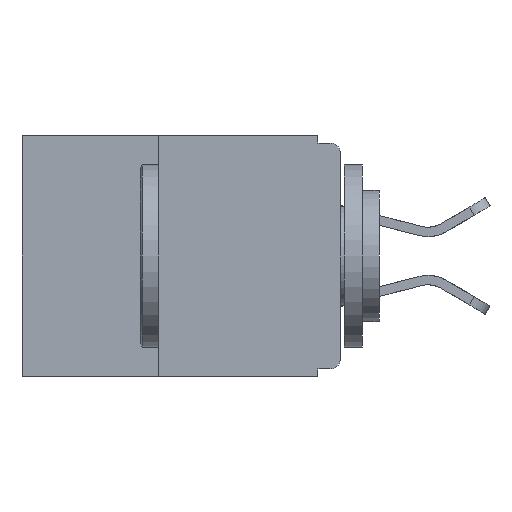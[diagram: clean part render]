
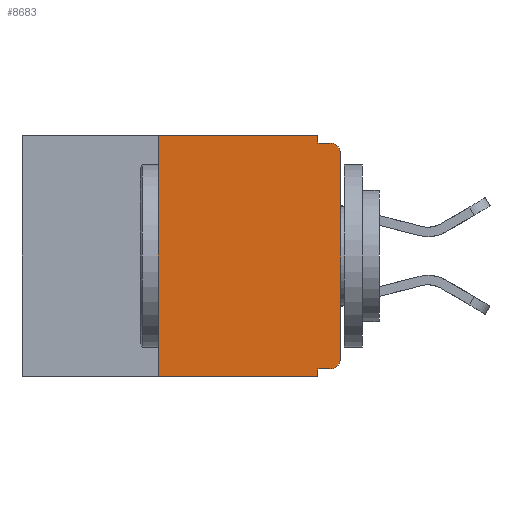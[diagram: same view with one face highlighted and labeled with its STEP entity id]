
A CAD part, left-side view. The second image highlights one B-rep face of the part: STEP entity #8683.
In plain terms, the highlighted planar face has unit normal (-1, 0, 0).
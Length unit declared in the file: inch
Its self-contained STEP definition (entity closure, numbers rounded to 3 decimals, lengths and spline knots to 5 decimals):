
#528 = EDGE_LOOP ( 'NONE', ( #21053, #15712, #7214, #2665, #1488, #900, #3362, #13361, #14241, #6404 ) ) ;
#668 = CARTESIAN_POINT ( 'NONE',  ( 0., 0.437, 0. ) ) ;
#900 = ORIENTED_EDGE ( 'NONE', *, *, #15830, .F. ) ;
#923 = EDGE_CURVE ( 'NONE', #12064, #20988, #22209, .T. ) ;
#1138 = CARTESIAN_POINT ( 'NONE',  ( 0., 0.031, -0.33 ) ) ;
#1488 = ORIENTED_EDGE ( 'NONE', *, *, #19813, .F. ) ;
#2294 = CARTESIAN_POINT ( 'NONE',  ( 0., 0., 0. ) ) ;
#2553 = PLANE ( 'NONE',  #15435 ) ;
#2558 = CARTESIAN_POINT ( 'NONE',  ( 0., 0.437, -0.33 ) ) ;
#2665 = ORIENTED_EDGE ( 'NONE', *, *, #14921, .F. ) ;
#2700 = DIRECTION ( 'NONE',  ( 0., 1., 0. ) ) ;
#2914 = EDGE_CURVE ( 'NONE', #7443, #11342, #14117, .T. ) ;
#3126 = CARTESIAN_POINT ( 'NONE',  ( 0., 0.031, 0. ) ) ;
#3134 = VECTOR ( 'NONE', #11284, 39.37008 ) ;
#3362 = ORIENTED_EDGE ( 'NONE', *, *, #923, .T. ) ;
#3385 = CARTESIAN_POINT ( 'NONE',  ( 0., 0., -0.305 ) ) ;
#3710 = VERTEX_POINT ( 'NONE', #20657 ) ;
#4427 = DIRECTION ( 'NONE',  ( 1., 0., 0. ) ) ;
#4460 = DIRECTION ( 'NONE',  ( 0., -1., 0. ) ) ;
#5360 = DIRECTION ( 'NONE',  ( -1., 0., 0. ) ) ;
#6025 = CARTESIAN_POINT ( 'NONE',  ( 0., 0.031, -0.32 ) ) ;
#6277 = EDGE_CURVE ( 'NONE', #6686, #22608, #18456, .T. ) ;
#6404 = ORIENTED_EDGE ( 'NONE', *, *, #2914, .T. ) ;
#6686 = VERTEX_POINT ( 'NONE', #11819 ) ;
#6876 = DIRECTION ( 'NONE',  ( 0., -1., 0. ) ) ;
#7000 = VERTEX_POINT ( 'NONE', #19838 ) ;
#7214 = ORIENTED_EDGE ( 'NONE', *, *, #22752, .F. ) ;
#7427 = VERTEX_POINT ( 'NONE', #3126 ) ;
#7443 = VERTEX_POINT ( 'NONE', #17680 ) ;
#8442 = DIRECTION ( 'NONE',  ( 0., 0., -1. ) ) ;
#8683 = ADVANCED_FACE ( 'NONE', ( #13807 ), #2553, .F. ) ;
#9443 = VECTOR ( 'NONE', #4460, 39.37008 ) ;
#9627 = AXIS2_PLACEMENT_3D ( 'NONE', #10300, #10303, #9845 ) ;
#9845 = DIRECTION ( 'NONE',  ( 0., 0., -1. ) ) ;
#10051 = VECTOR ( 'NONE', #22029, 39.37008 ) ;
#10216 = EDGE_CURVE ( 'NONE', #15869, #20988, #15130, .T. ) ;
#10300 = CARTESIAN_POINT ( 'NONE',  ( 0., 0.015, -0.305 ) ) ;
#10303 = DIRECTION ( 'NONE',  ( -1., 0., 0. ) ) ;
#10342 = VECTOR ( 'NONE', #12413, 39.37008 ) ;
#10482 = EDGE_CURVE ( 'NONE', #11342, #6686, #13716, .T. ) ;
#10823 = CARTESIAN_POINT ( 'NONE',  ( 0., 0.25, -0.33 ) ) ;
#11276 = VECTOR ( 'NONE', #6876, 39.37008 ) ;
#11284 = DIRECTION ( 'NONE',  ( 0., -1., 0. ) ) ;
#11342 = VERTEX_POINT ( 'NONE', #3385 ) ;
#11819 = CARTESIAN_POINT ( 'NONE',  ( 0., 0., -0.025 ) ) ;
#12064 = VERTEX_POINT ( 'NONE', #10823 ) ;
#12413 = DIRECTION ( 'NONE',  ( 0., 0., -1. ) ) ;
#13361 = ORIENTED_EDGE ( 'NONE', *, *, #10216, .F. ) ;
#13510 = CARTESIAN_POINT ( 'NONE',  ( 0., 0., -0.32 ) ) ;
#13716 = LINE ( 'NONE', #2294, #10051 ) ;
#13807 = FACE_OUTER_BOUND ( 'NONE', #528, .T. ) ;
#14117 = CIRCLE ( 'NONE', #9627, 0.015 ) ;
#14241 = ORIENTED_EDGE ( 'NONE', *, *, #19167, .F. ) ;
#14802 = LINE ( 'NONE', #17084, #9443 ) ;
#14906 = VECTOR ( 'NONE', #2700, 39.37008 ) ;
#14921 = EDGE_CURVE ( 'NONE', #7427, #7000, #16755, .T. ) ;
#15130 = LINE ( 'NONE', #21285, #10342 ) ;
#15435 = AXIS2_PLACEMENT_3D ( 'NONE', #668, #4427, #17047 ) ;
#15454 = LINE ( 'NONE', #13510, #14906 ) ;
#15465 = CARTESIAN_POINT ( 'NONE',  ( 0., 0.015, -0.01 ) ) ;
#15712 = ORIENTED_EDGE ( 'NONE', *, *, #6277, .T. ) ;
#15830 = EDGE_CURVE ( 'NONE', #12064, #3710, #20603, .T. ) ;
#15869 = VERTEX_POINT ( 'NONE', #6025 ) ;
#15895 = VECTOR ( 'NONE', #16661, 39.37008 ) ;
#16047 = LINE ( 'NONE', #21114, #11276 ) ;
#16147 = CARTESIAN_POINT ( 'NONE',  ( 0., 0.015, -0.025 ) ) ;
#16661 = DIRECTION ( 'NONE',  ( 0., 0., 1. ) ) ;
#16755 = LINE ( 'NONE', #17480, #20892 ) ;
#17047 = DIRECTION ( 'NONE',  ( 0., 0., -1. ) ) ;
#17084 = CARTESIAN_POINT ( 'NONE',  ( 0., 0.437, 0. ) ) ;
#17480 = CARTESIAN_POINT ( 'NONE',  ( 0., 0.031, 0. ) ) ;
#17680 = CARTESIAN_POINT ( 'NONE',  ( 0., 0.015, -0.32 ) ) ;
#17952 = DIRECTION ( 'NONE',  ( 0., 0., -1. ) ) ;
#18456 = CIRCLE ( 'NONE', #18968, 0.015 ) ;
#18968 = AXIS2_PLACEMENT_3D ( 'NONE', #16147, #5360, #17952 ) ;
#19167 = EDGE_CURVE ( 'NONE', #7443, #15869, #15454, .T. ) ;
#19813 = EDGE_CURVE ( 'NONE', #3710, #7427, #14802, .T. ) ;
#19838 = CARTESIAN_POINT ( 'NONE',  ( 0., 0.031, -0.01 ) ) ;
#20137 = CARTESIAN_POINT ( 'NONE',  ( 0., 0.25, -0.33 ) ) ;
#20603 = LINE ( 'NONE', #20137, #15895 ) ;
#20657 = CARTESIAN_POINT ( 'NONE',  ( 0., 0.25, 0. ) ) ;
#20892 = VECTOR ( 'NONE', #8442, 39.37008 ) ;
#20988 = VERTEX_POINT ( 'NONE', #1138 ) ;
#21053 = ORIENTED_EDGE ( 'NONE', *, *, #10482, .T. ) ;
#21114 = CARTESIAN_POINT ( 'NONE',  ( 0., 0., -0.01 ) ) ;
#21285 = CARTESIAN_POINT ( 'NONE',  ( 0., 0.031, -0.33 ) ) ;
#22029 = DIRECTION ( 'NONE',  ( 0., 0., 1. ) ) ;
#22209 = LINE ( 'NONE', #2558, #3134 ) ;
#22608 = VERTEX_POINT ( 'NONE', #15465 ) ;
#22752 = EDGE_CURVE ( 'NONE', #7000, #22608, #16047, .T. ) ;
